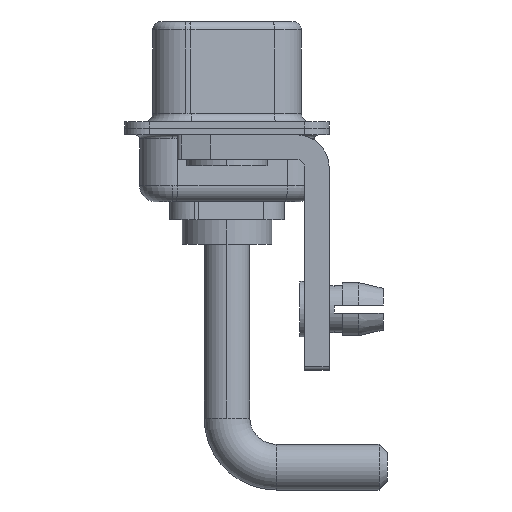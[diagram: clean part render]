
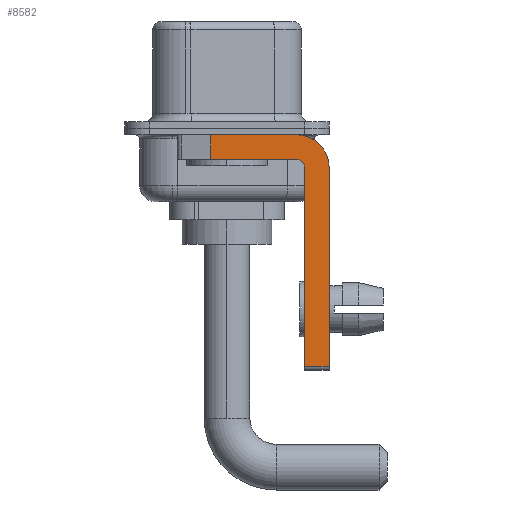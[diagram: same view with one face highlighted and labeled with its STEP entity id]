
A CAD part, left-side view. The second image highlights one B-rep face of the part: STEP entity #8582.
In plain terms, the highlighted planar face has unit normal (-1, 0, 0).
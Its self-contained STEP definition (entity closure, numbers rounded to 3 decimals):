
#465 = ORIENTED_EDGE ( 'NONE', *, *, #11182, .T. ) ;
#806 = VECTOR ( 'NONE', #16978, 1000. ) ;
#953 = DIRECTION ( 'NONE',  ( 0., 0., 1. ) ) ;
#1066 = AXIS2_PLACEMENT_3D ( 'NONE', #16341, #9112, #13356 ) ;
#1403 = VERTEX_POINT ( 'NONE', #13952 ) ;
#1942 = LINE ( 'NONE', #9019, #9728 ) ;
#2004 = VECTOR ( 'NONE', #4585, 1000. ) ;
#2092 = CARTESIAN_POINT ( 'NONE',  ( -2.9, 0.978, -0.4 ) ) ;
#2129 = DIRECTION ( 'NONE',  ( 0., -1., 0. ) ) ;
#2302 = DIRECTION ( 'NONE',  ( 0., 1., 0. ) ) ;
#3038 = ORIENTED_EDGE ( 'NONE', *, *, #6934, .F. ) ;
#3201 = VERTEX_POINT ( 'NONE', #10427 ) ;
#3557 = CARTESIAN_POINT ( 'NONE',  ( -2.9, -4.25, -1.9 ) ) ;
#3907 = DIRECTION ( 'NONE',  ( 0., 0., -1. ) ) ;
#4071 = DIRECTION ( 'NONE',  ( -1., 0., 0. ) ) ;
#4585 = DIRECTION ( 'NONE',  ( 0., 0., -1. ) ) ;
#4851 = AXIS2_PLACEMENT_3D ( 'NONE', #16904, #4071, #8371 ) ;
#5635 = CARTESIAN_POINT ( 'NONE',  ( -2.9, 3., -0.4 ) ) ;
#5763 = CARTESIAN_POINT ( 'NONE',  ( -2.9, -4.75, -2.4 ) ) ;
#5821 = EDGE_CURVE ( 'NONE', #1403, #3201, #6382, .T. ) ;
#6260 = VERTEX_POINT ( 'NONE', #17451 ) ;
#6337 = PLANE ( 'NONE',  #1066 ) ;
#6382 = LINE ( 'NONE', #12080, #14080 ) ;
#6934 = EDGE_CURVE ( 'NONE', #9740, #12670, #13582, .T. ) ;
#7009 = CARTESIAN_POINT ( 'NONE',  ( -2.9, 0.978, -1.9 ) ) ;
#7079 = ORIENTED_EDGE ( 'NONE', *, *, #13328, .T. ) ;
#7113 = ORIENTED_EDGE ( 'NONE', *, *, #7437, .F. ) ;
#7144 = VERTEX_POINT ( 'NONE', #17673 ) ;
#7354 = ORIENTED_EDGE ( 'NONE', *, *, #14797, .F. ) ;
#7437 = EDGE_CURVE ( 'NONE', #12670, #15489, #9315, .T. ) ;
#8371 = DIRECTION ( 'NONE',  ( 0., 0., 1. ) ) ;
#8565 = EDGE_CURVE ( 'NONE', #15489, #6260, #15122, .T. ) ;
#8582 = ADVANCED_FACE ( 'NONE', ( #14760 ), #6337, .F. ) ;
#8798 = EDGE_LOOP ( 'NONE', ( #12171, #465, #14763, #7113, #3038, #7079, #10263, #7354 ) ) ;
#9019 = CARTESIAN_POINT ( 'NONE',  ( -2.9, -4.25, -14.55 ) ) ;
#9112 = DIRECTION ( 'NONE',  ( 1., 0., 0. ) ) ;
#9315 = CIRCLE ( 'NONE', #4851, 0.5 ) ;
#9385 = CARTESIAN_POINT ( 'NONE',  ( -2.9, -4.25, -1.9 ) ) ;
#9502 = DIRECTION ( 'NONE',  ( 1., 0., 0. ) ) ;
#9728 = VECTOR ( 'NONE', #2129, 1000. ) ;
#9740 = VERTEX_POINT ( 'NONE', #17130 ) ;
#10068 = CIRCLE ( 'NONE', #11575, 2. ) ;
#10263 = ORIENTED_EDGE ( 'NONE', *, *, #5821, .F. ) ;
#10427 = CARTESIAN_POINT ( 'NONE',  ( -2.9, -6.25, -14.55 ) ) ;
#11182 = EDGE_CURVE ( 'NONE', #17258, #6260, #15920, .T. ) ;
#11575 = AXIS2_PLACEMENT_3D ( 'NONE', #16731, #9502, #3907 ) ;
#12080 = CARTESIAN_POINT ( 'NONE',  ( -2.9, -6.25, -2.4 ) ) ;
#12171 = ORIENTED_EDGE ( 'NONE', *, *, #13549, .F. ) ;
#12670 = VERTEX_POINT ( 'NONE', #5763 ) ;
#12943 = LINE ( 'NONE', #5635, #806 ) ;
#13328 = EDGE_CURVE ( 'NONE', #9740, #3201, #1942, .T. ) ;
#13356 = DIRECTION ( 'NONE',  ( 0., 0., -1. ) ) ;
#13549 = EDGE_CURVE ( 'NONE', #17258, #7144, #12943, .T. ) ;
#13582 = LINE ( 'NONE', #17871, #17099 ) ;
#13952 = CARTESIAN_POINT ( 'NONE',  ( -2.9, -6.25, -2.4 ) ) ;
#14080 = VECTOR ( 'NONE', #17794, 1000. ) ;
#14760 = FACE_OUTER_BOUND ( 'NONE', #8798, .T. ) ;
#14763 = ORIENTED_EDGE ( 'NONE', *, *, #8565, .F. ) ;
#14797 = EDGE_CURVE ( 'NONE', #7144, #1403, #10068, .T. ) ;
#15122 = LINE ( 'NONE', #9385, #15400 ) ;
#15400 = VECTOR ( 'NONE', #2302, 1000. ) ;
#15489 = VERTEX_POINT ( 'NONE', #3557 ) ;
#15920 = LINE ( 'NONE', #7009, #2004 ) ;
#16341 = CARTESIAN_POINT ( 'NONE',  ( -2.9, -4.25, -2.4 ) ) ;
#16731 = CARTESIAN_POINT ( 'NONE',  ( -2.9, -4.25, -2.4 ) ) ;
#16904 = CARTESIAN_POINT ( 'NONE',  ( -2.9, -4.25, -2.4 ) ) ;
#16978 = DIRECTION ( 'NONE',  ( 0., -1., 0. ) ) ;
#17099 = VECTOR ( 'NONE', #953, 1000. ) ;
#17130 = CARTESIAN_POINT ( 'NONE',  ( -2.9, -4.75, -14.55 ) ) ;
#17258 = VERTEX_POINT ( 'NONE', #2092 ) ;
#17451 = CARTESIAN_POINT ( 'NONE',  ( -2.9, 0.978, -1.9 ) ) ;
#17673 = CARTESIAN_POINT ( 'NONE',  ( -2.9, -4.25, -0.4 ) ) ;
#17794 = DIRECTION ( 'NONE',  ( 0., 0., -1. ) ) ;
#17871 = CARTESIAN_POINT ( 'NONE',  ( -2.9, -4.75, -14.8 ) ) ;
